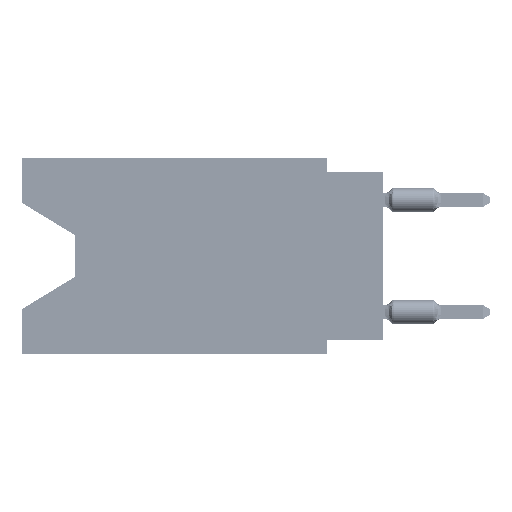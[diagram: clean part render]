
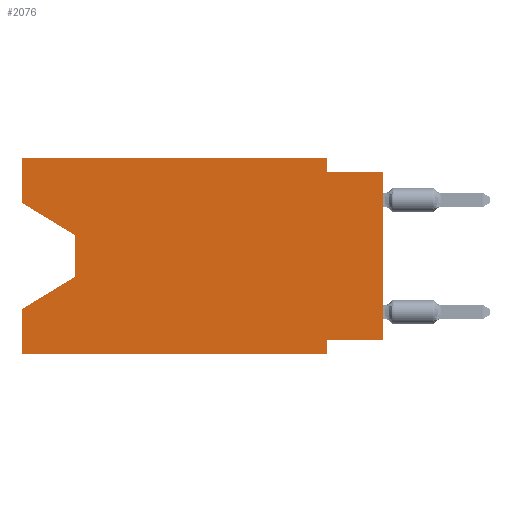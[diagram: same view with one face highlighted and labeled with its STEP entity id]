
A CAD part, left-side view. The second image highlights one B-rep face of the part: STEP entity #2076.
In plain terms, the highlighted planar face has unit normal (-1, 0, 0).
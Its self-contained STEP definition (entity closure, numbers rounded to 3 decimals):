
#725 = VECTOR ( 'NONE', #99429, 1000. ) ;
#830 = LINE ( 'NONE', #82215, #19877 ) ;
#856 = CARTESIAN_POINT ( 'NONE',  ( 0., 16.383, -2.038 ) ) ;
#1113 = LINE ( 'NONE', #27256, #68175 ) ;
#1864 = LINE ( 'NONE', #47580, #88716 ) ;
#2076 = ADVANCED_FACE ( 'NONE', ( #57029 ), #19617, .F. ) ;
#8509 = EDGE_CURVE ( 'NONE', #93725, #102482, #90650, .T. ) ;
#8907 = EDGE_CURVE ( 'NONE', #97340, #70897, #91095, .T. ) ;
#9149 = CARTESIAN_POINT ( 'NONE',  ( 0., 16.383, 0. ) ) ;
#9258 = ORIENTED_EDGE ( 'NONE', *, *, #77725, .T. ) ;
#10216 = EDGE_CURVE ( 'NONE', #22271, #102482, #830, .T. ) ;
#13643 = VECTOR ( 'NONE', #82992, 1000. ) ;
#16006 = CARTESIAN_POINT ( 'NONE',  ( 0., 0., -8.255 ) ) ;
#16617 = DIRECTION ( 'NONE',  ( 0., 0., -1. ) ) ;
#17051 = CARTESIAN_POINT ( 'NONE',  ( 0., 16.383, -6.852 ) ) ;
#17598 = CARTESIAN_POINT ( 'NONE',  ( 0., 0., -0.635 ) ) ;
#18967 = VECTOR ( 'NONE', #86816, 1000. ) ;
#19242 = DIRECTION ( 'NONE',  ( 0., 0., 1. ) ) ;
#19617 = PLANE ( 'NONE',  #88559 ) ;
#19877 = VECTOR ( 'NONE', #19242, 1000. ) ;
#21019 = CARTESIAN_POINT ( 'NONE',  ( 0., 2.54, -8.255 ) ) ;
#22271 = VERTEX_POINT ( 'NONE', #107270 ) ;
#23727 = DIRECTION ( 'NONE',  ( 0., 1., 0. ) ) ;
#27256 = CARTESIAN_POINT ( 'NONE',  ( 0., 16.383, 0. ) ) ;
#27260 = VECTOR ( 'NONE', #37759, 1000. ) ;
#28929 = LINE ( 'NONE', #58011, #13643 ) ;
#32167 = LINE ( 'NONE', #79646, #18967 ) ;
#33545 = CARTESIAN_POINT ( 'NONE',  ( 0., 2.54, -8.89 ) ) ;
#34695 = EDGE_CURVE ( 'NONE', #98843, #87655, #107512, .T. ) ;
#35590 = CARTESIAN_POINT ( 'NONE',  ( 0., 13.97, -3.505 ) ) ;
#37335 = DIRECTION ( 'NONE',  ( 0., -1., 0. ) ) ;
#37759 = DIRECTION ( 'NONE',  ( 0., -1., 0. ) ) ;
#37966 = ORIENTED_EDGE ( 'NONE', *, *, #63835, .F. ) ;
#38009 = CARTESIAN_POINT ( 'NONE',  ( 0., 16.383, 0. ) ) ;
#40846 = ORIENTED_EDGE ( 'NONE', *, *, #41282, .F. ) ;
#41282 = EDGE_CURVE ( 'NONE', #70897, #113614, #1113, .T. ) ;
#42689 = EDGE_CURVE ( 'NONE', #72919, #90021, #111041, .T. ) ;
#43288 = ORIENTED_EDGE ( 'NONE', *, *, #8907, .F. ) ;
#45765 = ORIENTED_EDGE ( 'NONE', *, *, #71134, .F. ) ;
#47580 = CARTESIAN_POINT ( 'NONE',  ( 0., 2.54, 0. ) ) ;
#54355 = CARTESIAN_POINT ( 'NONE',  ( 0., 13.97, -3.505 ) ) ;
#57029 = FACE_OUTER_BOUND ( 'NONE', #96160, .T. ) ;
#58011 = CARTESIAN_POINT ( 'NONE',  ( 0., 16.383, -8.89 ) ) ;
#58876 = CARTESIAN_POINT ( 'NONE',  ( 0., 2.54, -0.635 ) ) ;
#59491 = LINE ( 'NONE', #112982, #115783 ) ;
#59681 = ORIENTED_EDGE ( 'NONE', *, *, #34695, .T. ) ;
#63453 = CARTESIAN_POINT ( 'NONE',  ( 0., 0., -0.635 ) ) ;
#63835 = EDGE_CURVE ( 'NONE', #76067, #96203, #59491, .T. ) ;
#64823 = CARTESIAN_POINT ( 'NONE',  ( 0., 16.383, 0. ) ) ;
#68175 = VECTOR ( 'NONE', #37335, 1000. ) ;
#69352 = ORIENTED_EDGE ( 'NONE', *, *, #10216, .T. ) ;
#70897 = VERTEX_POINT ( 'NONE', #64823 ) ;
#71134 = EDGE_CURVE ( 'NONE', #22271, #76067, #71237, .T. ) ;
#71237 = LINE ( 'NONE', #16006, #99838 ) ;
#71531 = ORIENTED_EDGE ( 'NONE', *, *, #73014, .F. ) ;
#72919 = VERTEX_POINT ( 'NONE', #96943 ) ;
#73014 = EDGE_CURVE ( 'NONE', #113614, #93725, #1864, .T. ) ;
#75106 = DIRECTION ( 'NONE',  ( 0., -0.855, -0.519 ) ) ;
#75912 = ORIENTED_EDGE ( 'NONE', *, *, #42689, .F. ) ;
#76067 = VERTEX_POINT ( 'NONE', #21019 ) ;
#76631 = VECTOR ( 'NONE', #16617, 1000. ) ;
#77725 = EDGE_CURVE ( 'NONE', #87655, #90021, #32167, .T. ) ;
#79132 = ORIENTED_EDGE ( 'NONE', *, *, #99592, .T. ) ;
#79294 = CARTESIAN_POINT ( 'NONE',  ( 0., 2.54, 0. ) ) ;
#79646 = CARTESIAN_POINT ( 'NONE',  ( 0., 13.97, -5.385 ) ) ;
#82215 = CARTESIAN_POINT ( 'NONE',  ( 0., 0., 0. ) ) ;
#82582 = DIRECTION ( 'NONE',  ( 0., 0., -1. ) ) ;
#82992 = DIRECTION ( 'NONE',  ( 0., -1., 0. ) ) ;
#84003 = LINE ( 'NONE', #856, #94129 ) ;
#86816 = DIRECTION ( 'NONE',  ( 0., 0.855, -0.519 ) ) ;
#87655 = VERTEX_POINT ( 'NONE', #110718 ) ;
#88559 = AXIS2_PLACEMENT_3D ( 'NONE', #38009, #102169, #82582 ) ;
#88716 = VECTOR ( 'NONE', #91566, 1000. ) ;
#90021 = VERTEX_POINT ( 'NONE', #17051 ) ;
#90650 = LINE ( 'NONE', #17598, #27260 ) ;
#91095 = LINE ( 'NONE', #9149, #725 ) ;
#91566 = DIRECTION ( 'NONE',  ( 0., 0., -1. ) ) ;
#92602 = CARTESIAN_POINT ( 'NONE',  ( 0., 16.383, 0. ) ) ;
#93725 = VERTEX_POINT ( 'NONE', #58876 ) ;
#94129 = VECTOR ( 'NONE', #75106, 1000. ) ;
#94347 = DIRECTION ( 'NONE',  ( 0., 0., 1. ) ) ;
#95711 = DIRECTION ( 'NONE',  ( 0., 0., -1. ) ) ;
#96160 = EDGE_LOOP ( 'NONE', ( #96328, #59681, #9258, #75912, #79132, #37966, #45765, #69352, #114595, #71531, #40846, #43288 ) ) ;
#96203 = VERTEX_POINT ( 'NONE', #33545 ) ;
#96328 = ORIENTED_EDGE ( 'NONE', *, *, #114878, .T. ) ;
#96943 = CARTESIAN_POINT ( 'NONE',  ( 0., 16.383, -8.89 ) ) ;
#97340 = VERTEX_POINT ( 'NONE', #101974 ) ;
#98843 = VERTEX_POINT ( 'NONE', #54355 ) ;
#99429 = DIRECTION ( 'NONE',  ( 0., 0., 1. ) ) ;
#99592 = EDGE_CURVE ( 'NONE', #72919, #96203, #28929, .T. ) ;
#99838 = VECTOR ( 'NONE', #23727, 1000. ) ;
#101974 = CARTESIAN_POINT ( 'NONE',  ( 0., 16.383, -2.038 ) ) ;
#102169 = DIRECTION ( 'NONE',  ( 1., 0., 0. ) ) ;
#102482 = VERTEX_POINT ( 'NONE', #63453 ) ;
#106325 = VECTOR ( 'NONE', #94347, 1000. ) ;
#107270 = CARTESIAN_POINT ( 'NONE',  ( 0., 0., -8.255 ) ) ;
#107512 = LINE ( 'NONE', #35590, #76631 ) ;
#110718 = CARTESIAN_POINT ( 'NONE',  ( 0., 13.97, -5.385 ) ) ;
#111041 = LINE ( 'NONE', #92602, #106325 ) ;
#112982 = CARTESIAN_POINT ( 'NONE',  ( 0., 2.54, -8.89 ) ) ;
#113614 = VERTEX_POINT ( 'NONE', #79294 ) ;
#114595 = ORIENTED_EDGE ( 'NONE', *, *, #8509, .F. ) ;
#114878 = EDGE_CURVE ( 'NONE', #97340, #98843, #84003, .T. ) ;
#115783 = VECTOR ( 'NONE', #95711, 1000. ) ;
